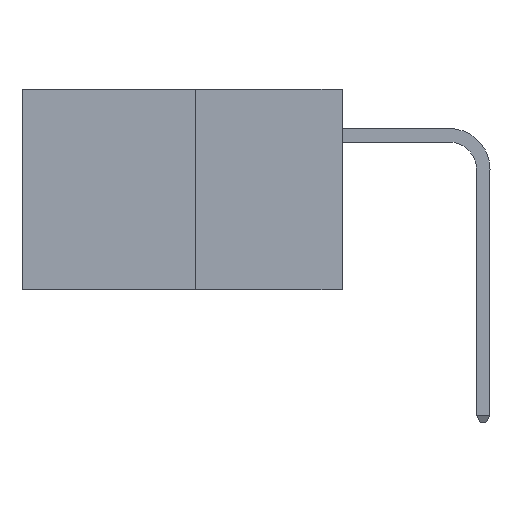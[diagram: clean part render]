
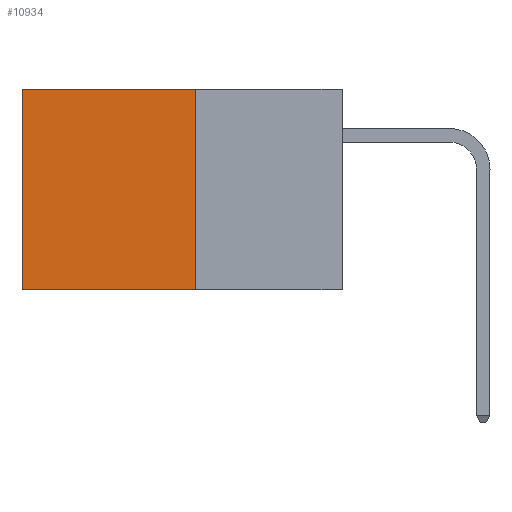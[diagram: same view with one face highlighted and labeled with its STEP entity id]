
A CAD part, left-side view. The second image highlights one B-rep face of the part: STEP entity #10934.
In plain terms, the highlighted planar face has unit normal (-1, 0, 0).
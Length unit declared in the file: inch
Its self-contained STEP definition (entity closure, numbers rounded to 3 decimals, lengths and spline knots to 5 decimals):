
#402 = VECTOR ( 'NONE', #20948, 39.37008 ) ;
#593 = CARTESIAN_POINT ( 'NONE',  ( 0.277, 0.59, 0. ) ) ;
#1035 = EDGE_CURVE ( 'NONE', #27476, #15731, #1991, .T. ) ;
#1073 = ORIENTED_EDGE ( 'NONE', *, *, #12796, .T. ) ;
#1991 = LINE ( 'NONE', #20925, #402 ) ;
#2351 = CARTESIAN_POINT ( 'NONE',  ( 0.277, 0.59, -0.37 ) ) ;
#2469 = ORIENTED_EDGE ( 'NONE', *, *, #31019, .F. ) ;
#3845 = DIRECTION ( 'NONE',  ( 0., 0., -1. ) ) ;
#4020 = DIRECTION ( 'NONE',  ( 1., 0., 0. ) ) ;
#4078 = LINE ( 'NONE', #26519, #11250 ) ;
#4321 = VERTEX_POINT ( 'NONE', #15831 ) ;
#4366 = PLANE ( 'NONE',  #31003 ) ;
#7114 = VECTOR ( 'NONE', #23888, 39.37008 ) ;
#7130 = EDGE_CURVE ( 'NONE', #4321, #15731, #28986, .T. ) ;
#8353 = CARTESIAN_POINT ( 'NONE',  ( 0.277, 0.27, 0. ) ) ;
#10934 = ADVANCED_FACE ( 'NONE', ( #17969 ), #4366, .F. ) ;
#11250 = VECTOR ( 'NONE', #24004, 39.37008 ) ;
#12796 = EDGE_CURVE ( 'NONE', #26858, #27476, #25021, .T. ) ;
#15731 = VERTEX_POINT ( 'NONE', #2351 ) ;
#15831 = CARTESIAN_POINT ( 'NONE',  ( 0.277, 0.27, -0.37 ) ) ;
#17969 = FACE_OUTER_BOUND ( 'NONE', #26512, .T. ) ;
#18210 = VECTOR ( 'NONE', #29259, 39.37008 ) ;
#19177 = CARTESIAN_POINT ( 'NONE',  ( 0.277, 0.27, 0. ) ) ;
#19211 = ORIENTED_EDGE ( 'NONE', *, *, #1035, .T. ) ;
#20925 = CARTESIAN_POINT ( 'NONE',  ( 0.277, 0.59, -0.37 ) ) ;
#20948 = DIRECTION ( 'NONE',  ( 0., 0., -1. ) ) ;
#22784 = CARTESIAN_POINT ( 'NONE',  ( 0.277, 0.27, -0.37 ) ) ;
#23888 = DIRECTION ( 'NONE',  ( 0., 1., 0. ) ) ;
#24004 = DIRECTION ( 'NONE',  ( 0., 0., -1. ) ) ;
#25021 = LINE ( 'NONE', #19177, #18210 ) ;
#25417 = CARTESIAN_POINT ( 'NONE',  ( 0.277, 0.27, -0.37 ) ) ;
#26512 = EDGE_LOOP ( 'NONE', ( #19211, #29168, #2469, #1073 ) ) ;
#26519 = CARTESIAN_POINT ( 'NONE',  ( 0.277, 0.27, -0.37 ) ) ;
#26858 = VERTEX_POINT ( 'NONE', #8353 ) ;
#27476 = VERTEX_POINT ( 'NONE', #593 ) ;
#28986 = LINE ( 'NONE', #25417, #7114 ) ;
#29168 = ORIENTED_EDGE ( 'NONE', *, *, #7130, .F. ) ;
#29259 = DIRECTION ( 'NONE',  ( 0., 1., 0. ) ) ;
#31003 = AXIS2_PLACEMENT_3D ( 'NONE', #22784, #4020, #3845 ) ;
#31019 = EDGE_CURVE ( 'NONE', #26858, #4321, #4078, .T. ) ;
